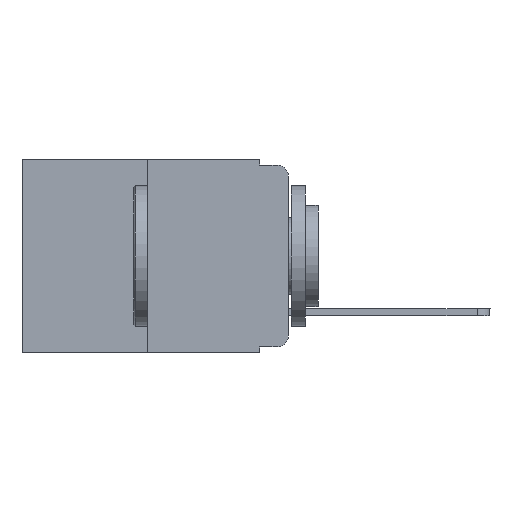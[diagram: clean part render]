
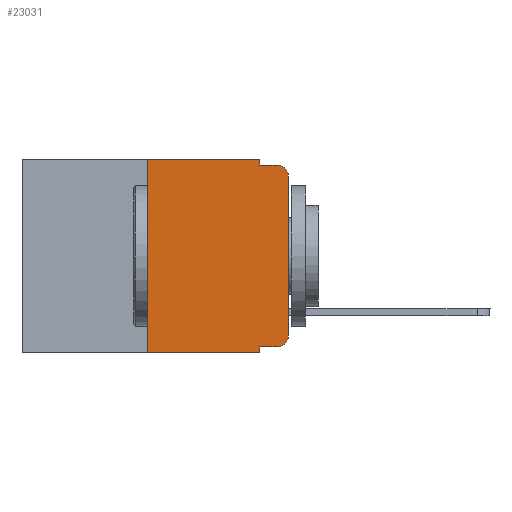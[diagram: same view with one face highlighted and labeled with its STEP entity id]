
A CAD part, left-side view. The second image highlights one B-rep face of the part: STEP entity #23031.
In plain terms, the highlighted planar face has unit normal (-1, 0, 0).
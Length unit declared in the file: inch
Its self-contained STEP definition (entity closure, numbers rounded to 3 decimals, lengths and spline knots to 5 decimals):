
#339 = LINE ( 'NONE', #20947, #21728 ) ;
#424 = ORIENTED_EDGE ( 'NONE', *, *, #18232, .F. ) ;
#678 = CARTESIAN_POINT ( 'NONE',  ( 0., 0., 0. ) ) ;
#864 = ORIENTED_EDGE ( 'NONE', *, *, #13529, .F. ) ;
#1765 = VECTOR ( 'NONE', #12395, 39.37008 ) ;
#1949 = CARTESIAN_POINT ( 'NONE',  ( 0., 0.02, -0.03 ) ) ;
#2026 = EDGE_CURVE ( 'NONE', #20861, #17309, #21938, .T. ) ;
#2132 = VERTEX_POINT ( 'NONE', #15007 ) ;
#2558 = EDGE_CURVE ( 'NONE', #20231, #14136, #339, .T. ) ;
#2729 = EDGE_CURVE ( 'NONE', #12726, #10205, #4404, .T. ) ;
#3118 = CARTESIAN_POINT ( 'NONE',  ( 0., 0.25, 0. ) ) ;
#3213 = CARTESIAN_POINT ( 'NONE',  ( 0., 0., -0.313 ) ) ;
#3407 = CARTESIAN_POINT ( 'NONE',  ( 0., 0.02, -0.313 ) ) ;
#3442 = DIRECTION ( 'NONE',  ( 0., 0., -1. ) ) ;
#3739 = EDGE_CURVE ( 'NONE', #17309, #20739, #15268, .T. ) ;
#3838 = VECTOR ( 'NONE', #16670, 39.37008 ) ;
#4404 = LINE ( 'NONE', #678, #3838 ) ;
#5138 = EDGE_LOOP ( 'NONE', ( #5295, #9647, #864, #11286, #22312, #18215, #19771, #424, #21588, #12841 ) ) ;
#5274 = CIRCLE ( 'NONE', #6006, 0.02 ) ;
#5295 = ORIENTED_EDGE ( 'NONE', *, *, #2729, .T. ) ;
#5380 = CARTESIAN_POINT ( 'NONE',  ( 0., 0.473, -0.343 ) ) ;
#5446 = CARTESIAN_POINT ( 'NONE',  ( 0., 0.473, 0. ) ) ;
#5951 = CARTESIAN_POINT ( 'NONE',  ( 0., 0.25, 0. ) ) ;
#6006 = AXIS2_PLACEMENT_3D ( 'NONE', #3407, #22814, #6764 ) ;
#6764 = DIRECTION ( 'NONE',  ( 0., 0., -1. ) ) ;
#7159 = CARTESIAN_POINT ( 'NONE',  ( 0., 0.02, -0.333 ) ) ;
#7567 = LINE ( 'NONE', #5951, #21759 ) ;
#8201 = CARTESIAN_POINT ( 'NONE',  ( 0., 0., -0.03 ) ) ;
#8365 = CARTESIAN_POINT ( 'NONE',  ( 0., 0.051, -0.333 ) ) ;
#8663 = EDGE_CURVE ( 'NONE', #10205, #14015, #19608, .T. ) ;
#9036 = DIRECTION ( 'NONE',  ( 0., 0., -1. ) ) ;
#9647 = ORIENTED_EDGE ( 'NONE', *, *, #8663, .T. ) ;
#10205 = VERTEX_POINT ( 'NONE', #8201 ) ;
#10772 = FACE_OUTER_BOUND ( 'NONE', #5138, .T. ) ;
#10816 = DIRECTION ( 'NONE',  ( 0., -1., 0. ) ) ;
#11286 = ORIENTED_EDGE ( 'NONE', *, *, #3739, .F. ) ;
#11506 = AXIS2_PLACEMENT_3D ( 'NONE', #19324, #19444, #3442 ) ;
#11756 = CARTESIAN_POINT ( 'NONE',  ( 0., 0.051, 0. ) ) ;
#12395 = DIRECTION ( 'NONE',  ( 0., -1., 0. ) ) ;
#12726 = VERTEX_POINT ( 'NONE', #3213 ) ;
#12841 = ORIENTED_EDGE ( 'NONE', *, *, #17126, .T. ) ;
#12902 = VECTOR ( 'NONE', #18397, 39.37008 ) ;
#13107 = VECTOR ( 'NONE', #17161, 39.37008 ) ;
#13131 = LINE ( 'NONE', #18940, #12902 ) ;
#13529 = EDGE_CURVE ( 'NONE', #20739, #14015, #21007, .T. ) ;
#13933 = PLANE ( 'NONE',  #11506 ) ;
#14015 = VERTEX_POINT ( 'NONE', #15819 ) ;
#14136 = VERTEX_POINT ( 'NONE', #7159 ) ;
#15007 = CARTESIAN_POINT ( 'NONE',  ( 0., 0.25, -0.343 ) ) ;
#15268 = LINE ( 'NONE', #22432, #13107 ) ;
#15538 = DIRECTION ( 'NONE',  ( 0., -1., 0. ) ) ;
#15819 = CARTESIAN_POINT ( 'NONE',  ( 0., 0.02, -0.01 ) ) ;
#16670 = DIRECTION ( 'NONE',  ( 0., 0., 1. ) ) ;
#16883 = VERTEX_POINT ( 'NONE', #22459 ) ;
#17126 = EDGE_CURVE ( 'NONE', #14136, #12726, #5274, .T. ) ;
#17161 = DIRECTION ( 'NONE',  ( 0., 0., -1. ) ) ;
#17180 = EDGE_CURVE ( 'NONE', #2132, #20861, #7567, .T. ) ;
#17309 = VERTEX_POINT ( 'NONE', #11756 ) ;
#17616 = CARTESIAN_POINT ( 'NONE',  ( 0., 0.051, -0.01 ) ) ;
#17725 = DIRECTION ( 'NONE',  ( 0., -1., 0. ) ) ;
#17809 = VECTOR ( 'NONE', #10816, 39.37008 ) ;
#18215 = ORIENTED_EDGE ( 'NONE', *, *, #17180, .F. ) ;
#18232 = EDGE_CURVE ( 'NONE', #20231, #16883, #13131, .T. ) ;
#18397 = DIRECTION ( 'NONE',  ( 0., 0., -1. ) ) ;
#18940 = CARTESIAN_POINT ( 'NONE',  ( 0., 0.051, 0. ) ) ;
#19300 = LINE ( 'NONE', #5380, #1765 ) ;
#19324 = CARTESIAN_POINT ( 'NONE',  ( 0., 0.473, 0. ) ) ;
#19444 = DIRECTION ( 'NONE',  ( 1., 0., 0. ) ) ;
#19608 = CIRCLE ( 'NONE', #19997, 0.02 ) ;
#19771 = ORIENTED_EDGE ( 'NONE', *, *, #21157, .T. ) ;
#19997 = AXIS2_PLACEMENT_3D ( 'NONE', #1949, #21580, #9036 ) ;
#20231 = VERTEX_POINT ( 'NONE', #8365 ) ;
#20739 = VERTEX_POINT ( 'NONE', #22528 ) ;
#20861 = VERTEX_POINT ( 'NONE', #3118 ) ;
#20947 = CARTESIAN_POINT ( 'NONE',  ( 0., 0.051, -0.333 ) ) ;
#21007 = LINE ( 'NONE', #17616, #22369 ) ;
#21157 = EDGE_CURVE ( 'NONE', #2132, #16883, #19300, .T. ) ;
#21519 = DIRECTION ( 'NONE',  ( 0., 0., 1. ) ) ;
#21580 = DIRECTION ( 'NONE',  ( -1., 0., 0. ) ) ;
#21588 = ORIENTED_EDGE ( 'NONE', *, *, #2558, .T. ) ;
#21728 = VECTOR ( 'NONE', #15538, 39.37008 ) ;
#21759 = VECTOR ( 'NONE', #21519, 39.37008 ) ;
#21938 = LINE ( 'NONE', #5446, #17809 ) ;
#22312 = ORIENTED_EDGE ( 'NONE', *, *, #2026, .F. ) ;
#22369 = VECTOR ( 'NONE', #17725, 39.37008 ) ;
#22432 = CARTESIAN_POINT ( 'NONE',  ( 0., 0.051, 0. ) ) ;
#22459 = CARTESIAN_POINT ( 'NONE',  ( 0., 0.051, -0.343 ) ) ;
#22528 = CARTESIAN_POINT ( 'NONE',  ( 0., 0.051, -0.01 ) ) ;
#22814 = DIRECTION ( 'NONE',  ( -1., 0., 0. ) ) ;
#23031 = ADVANCED_FACE ( 'NONE', ( #10772 ), #13933, .F. ) ;
